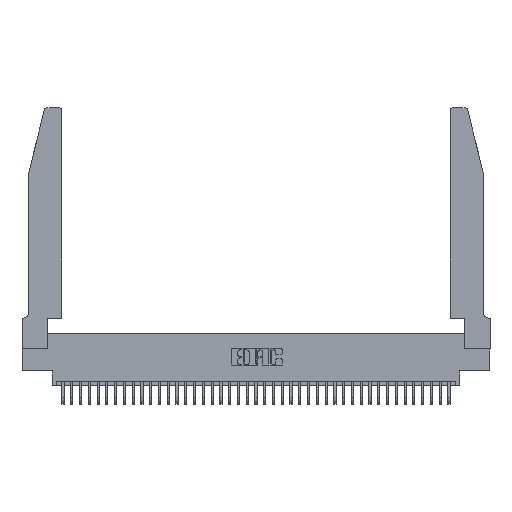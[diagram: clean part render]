
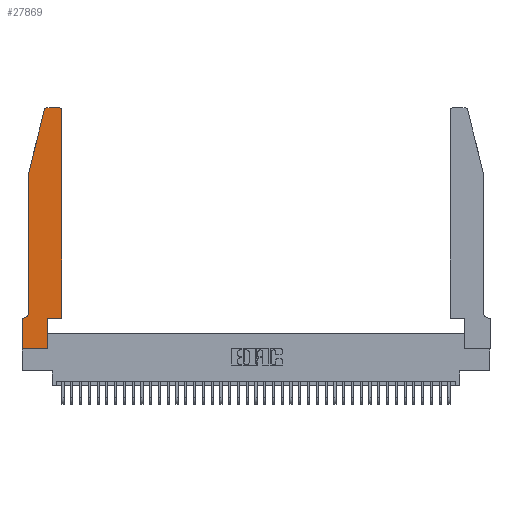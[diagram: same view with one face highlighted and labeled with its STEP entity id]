
A CAD part, top view. The second image highlights one B-rep face of the part: STEP entity #27869.
In plain terms, the highlighted planar face has unit normal (0, 0, 1).
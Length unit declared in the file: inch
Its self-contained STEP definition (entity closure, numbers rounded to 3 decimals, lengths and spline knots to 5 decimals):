
#463 = VERTEX_POINT ( 'NONE', #32271 ) ;
#530 = CARTESIAN_POINT ( 'NONE',  ( 0.4505, 0.35, 0.37 ) ) ;
#579 = CARTESIAN_POINT ( 'NONE',  ( 0., 0., 0.37 ) ) ;
#1798 = CARTESIAN_POINT ( 'NONE',  ( 0.4505, 2.72, 0.37 ) ) ;
#2057 = VERTEX_POINT ( 'NONE', #26478 ) ;
#2109 = PLANE ( 'NONE',  #12213 ) ;
#2562 = VECTOR ( 'NONE', #22916, 39.37008 ) ;
#2728 = VERTEX_POINT ( 'NONE', #34440 ) ;
#2802 = ORIENTED_EDGE ( 'NONE', *, *, #17035, .T. ) ;
#3864 = ORIENTED_EDGE ( 'NONE', *, *, #17743, .T. ) ;
#5168 = EDGE_CURVE ( 'NONE', #15824, #8086, #11947, .T. ) ;
#5519 = FACE_OUTER_BOUND ( 'NONE', #22415, .T. ) ;
#6799 = CARTESIAN_POINT ( 'NONE',  ( 0.4205, 2.72, 0.37 ) ) ;
#6840 = EDGE_CURVE ( 'NONE', #32349, #15824, #25252, .T. ) ;
#7616 = EDGE_CURVE ( 'NONE', #25377, #2728, #20718, .T. ) ;
#8086 = VERTEX_POINT ( 'NONE', #27969 ) ;
#8787 = DIRECTION ( 'NONE',  ( 1., 0., 0. ) ) ;
#8968 = DIRECTION ( 'NONE',  ( 0., 0., 1. ) ) ;
#10002 = CARTESIAN_POINT ( 'NONE',  ( 0., 0., 0.37 ) ) ;
#10710 = VECTOR ( 'NONE', #34096, 39.37008 ) ;
#11019 = DIRECTION ( 'NONE',  ( -1., 0., 0. ) ) ;
#11720 = CARTESIAN_POINT ( 'NONE',  ( 0.2865, 0.35, 0.37 ) ) ;
#11750 = DIRECTION ( 'NONE',  ( 0., 0., 1. ) ) ;
#11947 = LINE ( 'NONE', #11720, #30937 ) ;
#12121 = ORIENTED_EDGE ( 'NONE', *, *, #16714, .T. ) ;
#12143 = CIRCLE ( 'NONE', #13850, 0.03 ) ;
#12213 = AXIS2_PLACEMENT_3D ( 'NONE', #24731, #8968, #18326 ) ;
#12245 = VERTEX_POINT ( 'NONE', #41163 ) ;
#12578 = LINE ( 'NONE', #530, #2562 ) ;
#12685 = CIRCLE ( 'NONE', #37990, 0.07 ) ;
#13128 = EDGE_CURVE ( 'NONE', #2728, #463, #30239, .T. ) ;
#13223 = LINE ( 'NONE', #14121, #10710 ) ;
#13850 = AXIS2_PLACEMENT_3D ( 'NONE', #6799, #38900, #8787 ) ;
#13864 = CARTESIAN_POINT ( 'NONE',  ( 0., 0.35, 0.37 ) ) ;
#14121 = CARTESIAN_POINT ( 'NONE',  ( 0.4505, 0.35, 0.37 ) ) ;
#14759 = VECTOR ( 'NONE', #38990, 39.37008 ) ;
#15288 = VERTEX_POINT ( 'NONE', #13864 ) ;
#15824 = VERTEX_POINT ( 'NONE', #23238 ) ;
#16570 = EDGE_CURVE ( 'NONE', #15288, #32349, #22276, .T. ) ;
#16714 = EDGE_CURVE ( 'NONE', #34517, #38489, #13223, .T. ) ;
#16767 = LINE ( 'NONE', #26922, #36351 ) ;
#17035 = EDGE_CURVE ( 'NONE', #12245, #24254, #12685, .T. ) ;
#17063 = CARTESIAN_POINT ( 'NONE',  ( 0.0055, 0.42, 0.37 ) ) ;
#17743 = EDGE_CURVE ( 'NONE', #38489, #25377, #12143, .T. ) ;
#17897 = ORIENTED_EDGE ( 'NONE', *, *, #31213, .T. ) ;
#18326 = DIRECTION ( 'NONE',  ( 1., 0., 0. ) ) ;
#18684 = EDGE_CURVE ( 'NONE', #8086, #34517, #12578, .T. ) ;
#18725 = VECTOR ( 'NONE', #23497, 39.37008 ) ;
#19490 = LINE ( 'NONE', #30391, #28965 ) ;
#19801 = VECTOR ( 'NONE', #20162, 39.37008 ) ;
#20162 = DIRECTION ( 'NONE',  ( 0., -1., 0. ) ) ;
#20718 = LINE ( 'NONE', #22994, #18725 ) ;
#21385 = CARTESIAN_POINT ( 'NONE',  ( 0.4505, 0.35, 0.37 ) ) ;
#22004 = CARTESIAN_POINT ( 'NONE',  ( 0., 0., 0.37 ) ) ;
#22276 = LINE ( 'NONE', #579, #14759 ) ;
#22415 = EDGE_LOOP ( 'NONE', ( #30138, #30242, #25110, #17897, #2802, #29681, #23542, #34387, #27121, #25009, #12121, #3864 ) ) ;
#22509 = DIRECTION ( 'NONE',  ( 1., 0., 0. ) ) ;
#22916 = DIRECTION ( 'NONE',  ( 1., 0., 0. ) ) ;
#22994 = CARTESIAN_POINT ( 'NONE',  ( 0.2605, 2.75, 0.37 ) ) ;
#23238 = CARTESIAN_POINT ( 'NONE',  ( 0.2865, 0., 0.37 ) ) ;
#23497 = DIRECTION ( 'NONE',  ( -1., 0., 0. ) ) ;
#23542 = ORIENTED_EDGE ( 'NONE', *, *, #16570, .T. ) ;
#24254 = VERTEX_POINT ( 'NONE', #28222 ) ;
#24731 = CARTESIAN_POINT ( 'NONE',  ( 0., 0.35, 0.37 ) ) ;
#25009 = ORIENTED_EDGE ( 'NONE', *, *, #18684, .T. ) ;
#25062 = EDGE_CURVE ( 'NONE', #24254, #15288, #16767, .T. ) ;
#25110 = ORIENTED_EDGE ( 'NONE', *, *, #37154, .T. ) ;
#25252 = LINE ( 'NONE', #22004, #41359 ) ;
#25377 = VERTEX_POINT ( 'NONE', #32733 ) ;
#26478 = CARTESIAN_POINT ( 'NONE',  ( 0.0755, 2., 0.37 ) ) ;
#26922 = CARTESIAN_POINT ( 'NONE',  ( 0.0755, 0.35, 0.37 ) ) ;
#27093 = DIRECTION ( 'NONE',  ( 1., 0., 0. ) ) ;
#27121 = ORIENTED_EDGE ( 'NONE', *, *, #5168, .T. ) ;
#27869 = ADVANCED_FACE ( 'NONE', ( #5519 ), #2109, .T. ) ;
#27969 = CARTESIAN_POINT ( 'NONE',  ( 0.2865, 0.35, 0.37 ) ) ;
#28222 = CARTESIAN_POINT ( 'NONE',  ( 0.0055, 0.35, 0.37 ) ) ;
#28965 = VECTOR ( 'NONE', #30106, 39.37008 ) ;
#29021 = AXIS2_PLACEMENT_3D ( 'NONE', #30891, #11750, #27093 ) ;
#29681 = ORIENTED_EDGE ( 'NONE', *, *, #25062, .T. ) ;
#30106 = DIRECTION ( 'NONE',  ( -0.239, -0.971, 0. ) ) ;
#30138 = ORIENTED_EDGE ( 'NONE', *, *, #7616, .T. ) ;
#30239 = CIRCLE ( 'NONE', #29021, 0.03 ) ;
#30242 = ORIENTED_EDGE ( 'NONE', *, *, #13128, .T. ) ;
#30391 = CARTESIAN_POINT ( 'NONE',  ( 0.0755, 2., 0.37 ) ) ;
#30891 = CARTESIAN_POINT ( 'NONE',  ( 0.284, 2.72, 0.37 ) ) ;
#30937 = VECTOR ( 'NONE', #31146, 39.37008 ) ;
#31146 = DIRECTION ( 'NONE',  ( 0., 1., 0. ) ) ;
#31213 = EDGE_CURVE ( 'NONE', #2057, #12245, #34304, .T. ) ;
#32046 = CARTESIAN_POINT ( 'NONE',  ( 0.0755, 2., 0.37 ) ) ;
#32271 = CARTESIAN_POINT ( 'NONE',  ( 0.25487, 2.72718, 0.37 ) ) ;
#32349 = VERTEX_POINT ( 'NONE', #10002 ) ;
#32733 = CARTESIAN_POINT ( 'NONE',  ( 0.4205, 2.75, 0.37 ) ) ;
#34096 = DIRECTION ( 'NONE',  ( 0., 1., 0. ) ) ;
#34304 = LINE ( 'NONE', #32046, #19801 ) ;
#34387 = ORIENTED_EDGE ( 'NONE', *, *, #6840, .T. ) ;
#34440 = CARTESIAN_POINT ( 'NONE',  ( 0.284, 2.75, 0.37 ) ) ;
#34517 = VERTEX_POINT ( 'NONE', #21385 ) ;
#36351 = VECTOR ( 'NONE', #11019, 39.37008 ) ;
#36389 = DIRECTION ( 'NONE',  ( 0., 0., -1. ) ) ;
#37154 = EDGE_CURVE ( 'NONE', #463, #2057, #19490, .T. ) ;
#37990 = AXIS2_PLACEMENT_3D ( 'NONE', #17063, #36389, #39540 ) ;
#38489 = VERTEX_POINT ( 'NONE', #1798 ) ;
#38900 = DIRECTION ( 'NONE',  ( 0., 0., 1. ) ) ;
#38990 = DIRECTION ( 'NONE',  ( 0., -1., 0. ) ) ;
#39540 = DIRECTION ( 'NONE',  ( -1., 0., 0. ) ) ;
#41163 = CARTESIAN_POINT ( 'NONE',  ( 0.0755, 0.42, 0.37 ) ) ;
#41359 = VECTOR ( 'NONE', #22509, 39.37008 ) ;
